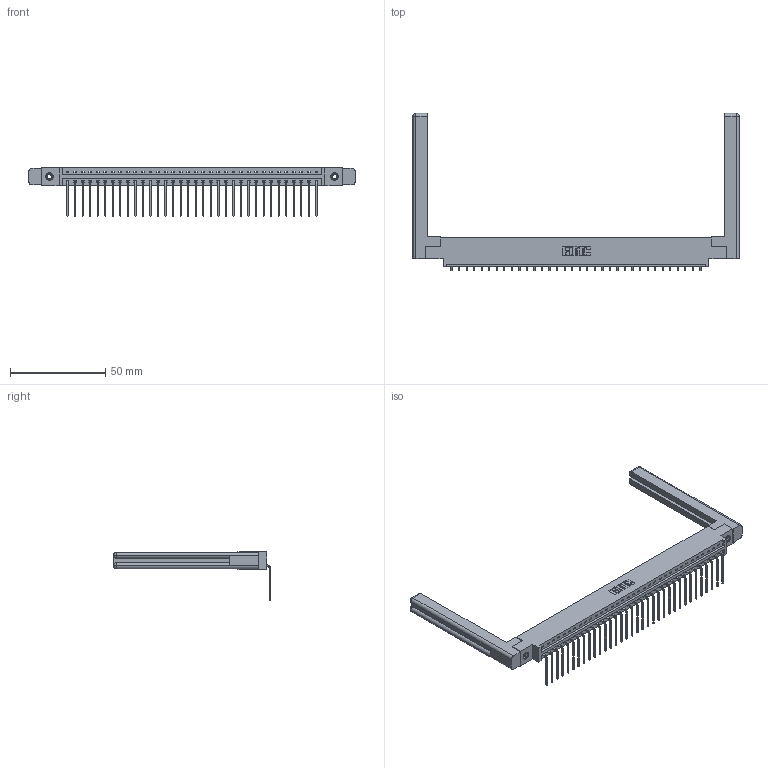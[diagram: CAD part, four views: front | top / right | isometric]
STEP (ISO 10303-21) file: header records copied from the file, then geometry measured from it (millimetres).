
FILE_DESCRIPTION (( 'STEP AP203' ), '1' );
FILE_NAME ('387-034-559-658.STEP', '2019-10-04T11:43:52', ( '' ), ( '' ), 'SwSTEP 2.0', 'SolidWorks 2016', '' );
FILE_SCHEMA (( 'CONFIG_CONTROL_DESIGN' ));
Length unit declared in the file: inch
Products named in the file (5): 345-250-001_345-250-001-102; 387-034-559-658; 345-292-001_558 559 Tail - 1; 337 Part_0.170 Offset - 0.156 Dia-TI; 307-220-058
Assembly tree (39 placements, depth 2):
  387-034-559-658
    337 Part_0.170 Offset - 0.156 Dia-TI
    345-292-001_558 559 Tail - 1  x34
    345-250-001_345-250-001-102  x2
    307-220-058  x2
Bounding box: 171.35 x 82.49 x 25.53 mm (x, y, z)
Volume: 24866.6 mm3; surface area: 24255.9 mm2
Topology: 39 solids, 39 shells, 2436 faces, 7273 edges, 4790 vertices
Faces by surface type: plane 1790, cylinder 622, cone 12, torus 12
Entity records: 29158 total; most frequent: CARTESIAN_POINT 5079, ORIENTED_EDGE 4988, DIRECTION 4310, EDGE_CURVE 2494, LINE 2318, VECTOR 2318, VERTEX_POINT 1654, AXIS2_PLACEMENT_3D 996
